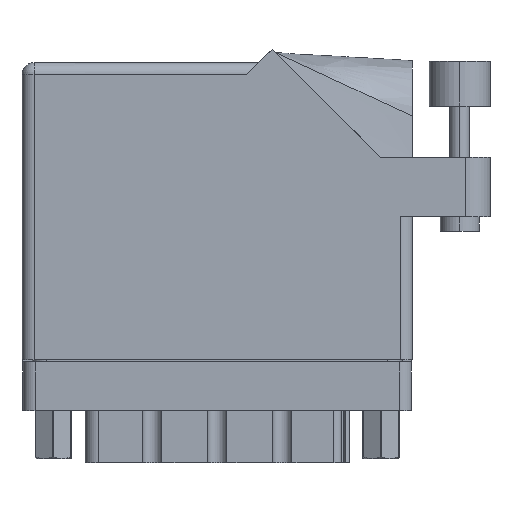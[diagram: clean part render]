
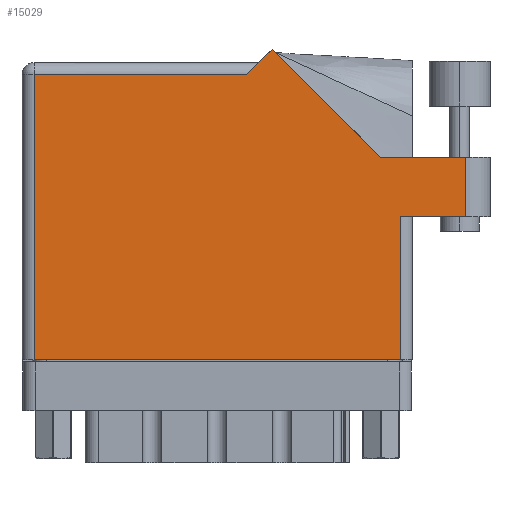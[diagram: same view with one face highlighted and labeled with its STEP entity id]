
A CAD part, front view. The second image highlights one B-rep face of the part: STEP entity #15029.
In plain terms, the highlighted face is planar.
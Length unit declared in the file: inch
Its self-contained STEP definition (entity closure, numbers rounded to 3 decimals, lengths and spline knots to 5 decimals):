
#42 = DIRECTION ( 'NONE',  ( -1., 0., 0. ) ) ;
#284 = DIRECTION ( 'NONE',  ( -1., 0., 0. ) ) ;
#354 = EDGE_CURVE ( 'NONE', #48803, #46922, #22740, .T. ) ;
#460 = ORIENTED_EDGE ( 'NONE', *, *, #37440, .T. ) ;
#3433 = ORIENTED_EDGE ( 'NONE', *, *, #18908, .T. ) ;
#3790 = LINE ( 'NONE', #23086, #16444 ) ;
#3987 = DIRECTION ( 'NONE',  ( 0., 0., -1. ) ) ;
#4360 = DIRECTION ( 'NONE',  ( -0.707, 0.707, 0. ) ) ;
#4517 = CARTESIAN_POINT ( 'NONE',  ( 2.01, 0.737, 0. ) ) ;
#4915 = ORIENTED_EDGE ( 'NONE', *, *, #21846, .T. ) ;
#5546 = DIRECTION ( 'NONE',  ( -0.707, -0.707, 0. ) ) ;
#5830 = CARTESIAN_POINT ( 'NONE',  ( 1.155, 1.468, 0. ) ) ;
#6389 = CARTESIAN_POINT ( 'NONE',  ( 2.285, 0.737, 0. ) ) ;
#6426 = CARTESIAN_POINT ( 'NONE',  ( 1.28771, 1.60071, 0. ) ) ;
#6694 = LINE ( 'NONE', #23084, #47095 ) ;
#7643 = LINE ( 'NONE', #4517, #44933 ) ;
#8109 = ORIENTED_EDGE ( 'NONE', *, *, #44008, .T. ) ;
#9346 = VECTOR ( 'NONE', #27869, 39.37008 ) ;
#10397 = EDGE_CURVE ( 'NONE', #11858, #11008, #32125, .T. ) ;
#11008 = VERTEX_POINT ( 'NONE', #5830 ) ;
#11858 = VERTEX_POINT ( 'NONE', #6426 ) ;
#13003 = ORIENTED_EDGE ( 'NONE', *, *, #10397, .T. ) ;
#13077 = CARTESIAN_POINT ( 'NONE',  ( 1.84442, 1.044, 0. ) ) ;
#13417 = AXIS2_PLACEMENT_3D ( 'NONE', #35051, #3987, #284 ) ;
#14568 = EDGE_CURVE ( 'NONE', #11008, #46502, #35210, .T. ) ;
#15029 = ADVANCED_FACE ( 'NONE', ( #24369 ), #15947, .F. ) ;
#15947 = PLANE ( 'NONE',  #13417 ) ;
#16444 = VECTOR ( 'NONE', #31609, 39.37008 ) ;
#18201 = CARTESIAN_POINT ( 'NONE',  ( 2.285, 1.044, 0. ) ) ;
#18908 = EDGE_CURVE ( 'NONE', #47944, #27673, #7643, .T. ) ;
#21675 = CARTESIAN_POINT ( 'NONE',  ( 1.948, 0., 0. ) ) ;
#21846 = EDGE_CURVE ( 'NONE', #43125, #31294, #6694, .T. ) ;
#22740 = LINE ( 'NONE', #30547, #29329 ) ;
#23084 = CARTESIAN_POINT ( 'NONE',  ( 2.41, 1.044, 0. ) ) ;
#23086 = CARTESIAN_POINT ( 'NONE',  ( 2.285, 1.044, 0. ) ) ;
#24183 = DIRECTION ( 'NONE',  ( -1., 0., 0. ) ) ;
#24263 = CARTESIAN_POINT ( 'NONE',  ( 1.948, 0.737, 0. ) ) ;
#24369 = FACE_OUTER_BOUND ( 'NONE', #27054, .T. ) ;
#24556 = DIRECTION ( 'NONE',  ( 0., -1., 0. ) ) ;
#26222 = VECTOR ( 'NONE', #24183, 39.37008 ) ;
#26722 = VECTOR ( 'NONE', #5546, 39.37008 ) ;
#26805 = EDGE_CURVE ( 'NONE', #31294, #11858, #31556, .T. ) ;
#27054 = EDGE_LOOP ( 'NONE', ( #3433, #460, #4915, #35882, #13003, #27301, #31613, #28398, #8109 ) ) ;
#27301 = ORIENTED_EDGE ( 'NONE', *, *, #14568, .T. ) ;
#27548 = CARTESIAN_POINT ( 'NONE',  ( 1.948, 0.737, 0. ) ) ;
#27673 = VERTEX_POINT ( 'NONE', #6389 ) ;
#27869 = DIRECTION ( 'NONE',  ( 0., 1., 0. ) ) ;
#28398 = ORIENTED_EDGE ( 'NONE', *, *, #354, .T. ) ;
#29329 = VECTOR ( 'NONE', #42184, 39.37008 ) ;
#30547 = CARTESIAN_POINT ( 'NONE',  ( 0., 0., 0. ) ) ;
#30777 = CARTESIAN_POINT ( 'NONE',  ( 0.062, 1.468, 0. ) ) ;
#31294 = VERTEX_POINT ( 'NONE', #13077 ) ;
#31403 = DIRECTION ( 'NONE',  ( 1., 0., 0. ) ) ;
#31556 = LINE ( 'NONE', #38481, #45463 ) ;
#31609 = DIRECTION ( 'NONE',  ( 0., 1., 0. ) ) ;
#31613 = ORIENTED_EDGE ( 'NONE', *, *, #48621, .T. ) ;
#31747 = CARTESIAN_POINT ( 'NONE',  ( 0., 1.468, 0. ) ) ;
#32125 = LINE ( 'NONE', #35636, #26722 ) ;
#35051 = CARTESIAN_POINT ( 'NONE',  ( 0., 1.53, 0. ) ) ;
#35210 = LINE ( 'NONE', #31747, #26222 ) ;
#35220 = LINE ( 'NONE', #27548, #9346 ) ;
#35619 = CARTESIAN_POINT ( 'NONE',  ( 0.062, 0., 0. ) ) ;
#35636 = CARTESIAN_POINT ( 'NONE',  ( 1.217, 1.53, 0. ) ) ;
#35882 = ORIENTED_EDGE ( 'NONE', *, *, #26805, .T. ) ;
#36678 = VECTOR ( 'NONE', #24556, 39.37008 ) ;
#36779 = CARTESIAN_POINT ( 'NONE',  ( 0.062, 0., 0. ) ) ;
#37440 = EDGE_CURVE ( 'NONE', #27673, #43125, #3790, .T. ) ;
#38481 = CARTESIAN_POINT ( 'NONE',  ( 1.84442, 1.044, 0. ) ) ;
#42184 = DIRECTION ( 'NONE',  ( 1., 0., 0. ) ) ;
#43125 = VERTEX_POINT ( 'NONE', #18201 ) ;
#44008 = EDGE_CURVE ( 'NONE', #46922, #47944, #35220, .T. ) ;
#44933 = VECTOR ( 'NONE', #31403, 39.37008 ) ;
#45139 = LINE ( 'NONE', #35619, #36678 ) ;
#45463 = VECTOR ( 'NONE', #4360, 39.37008 ) ;
#46502 = VERTEX_POINT ( 'NONE', #30777 ) ;
#46922 = VERTEX_POINT ( 'NONE', #21675 ) ;
#47095 = VECTOR ( 'NONE', #42, 39.37008 ) ;
#47944 = VERTEX_POINT ( 'NONE', #24263 ) ;
#48621 = EDGE_CURVE ( 'NONE', #46502, #48803, #45139, .T. ) ;
#48803 = VERTEX_POINT ( 'NONE', #36779 ) ;
